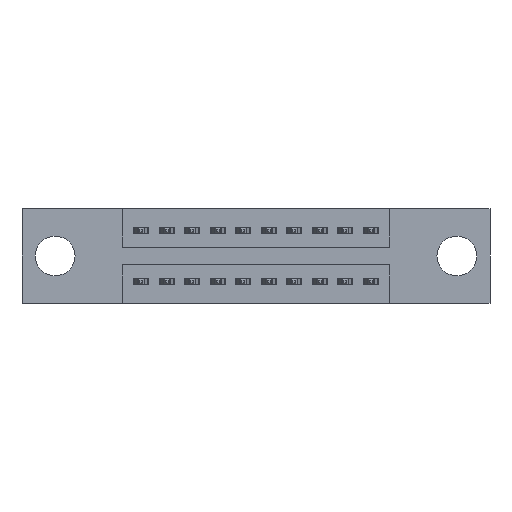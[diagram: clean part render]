
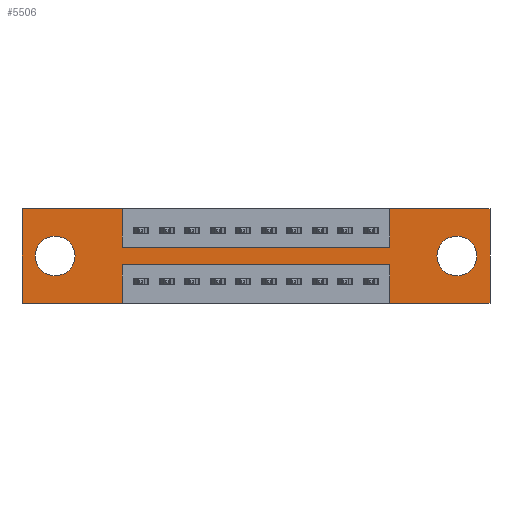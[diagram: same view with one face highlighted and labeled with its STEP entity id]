
A CAD part, front view. The second image highlights one B-rep face of the part: STEP entity #5506.
In plain terms, the highlighted planar face has unit normal (0, -1, 0).
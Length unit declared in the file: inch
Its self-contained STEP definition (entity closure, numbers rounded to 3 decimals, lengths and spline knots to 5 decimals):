
#204 = VERTEX_POINT ( 'NONE', #6562 ) ;
#367 = EDGE_LOOP ( 'NONE', ( #8075, #10543, #10820, #991, #1277, #11371, #1578, #11629, #4822, #7326, #10103, #7926 ) ) ;
#392 = VERTEX_POINT ( 'NONE', #11433 ) ;
#445 = EDGE_CURVE ( 'NONE', #9873, #9577, #7534, .T. ) ;
#560 = VERTEX_POINT ( 'NONE', #6616 ) ;
#700 = EDGE_CURVE ( 'NONE', #11317, #5010, #3963, .T. ) ;
#730 = VECTOR ( 'NONE', #9499, 39.37008 ) ;
#809 = DIRECTION ( 'NONE',  ( 1., 0., 0. ) ) ;
#852 = LINE ( 'NONE', #5624, #5449 ) ;
#991 = ORIENTED_EDGE ( 'NONE', *, *, #1927, .F. ) ;
#1004 = CIRCLE ( 'NONE', #9841, 0.078 ) ;
#1061 = VERTEX_POINT ( 'NONE', #1727 ) ;
#1115 = FACE_OUTER_BOUND ( 'NONE', #367, .T. ) ;
#1277 = ORIENTED_EDGE ( 'NONE', *, *, #700, .F. ) ;
#1292 = CARTESIAN_POINT ( 'NONE',  ( 1.705, 0., -0.185 ) ) ;
#1464 = VECTOR ( 'NONE', #4705, 39.37008 ) ;
#1578 = ORIENTED_EDGE ( 'NONE', *, *, #9920, .F. ) ;
#1727 = CARTESIAN_POINT ( 'NONE',  ( 1.4425, 0., -0.22 ) ) ;
#1927 = EDGE_CURVE ( 'NONE', #5010, #10494, #2683, .T. ) ;
#2093 = DIRECTION ( 'NONE',  ( -1., 0., 0. ) ) ;
#2102 = LINE ( 'NONE', #11151, #9720 ) ;
#2285 = DIRECTION ( 'NONE',  ( 0., 0., -1. ) ) ;
#2384 = CARTESIAN_POINT ( 'NONE',  ( 1.705, 0., -0.185 ) ) ;
#2396 = EDGE_CURVE ( 'NONE', #2643, #392, #3286, .T. ) ;
#2584 = AXIS2_PLACEMENT_3D ( 'NONE', #8527, #2786, #9447 ) ;
#2643 = VERTEX_POINT ( 'NONE', #4557 ) ;
#2674 = CARTESIAN_POINT ( 'NONE',  ( 1.705, 0., -0.263 ) ) ;
#2683 = LINE ( 'NONE', #3256, #9992 ) ;
#2703 = EDGE_CURVE ( 'NONE', #204, #11317, #852, .T. ) ;
#2755 = CARTESIAN_POINT ( 'NONE',  ( 1.4425, 0., 0. ) ) ;
#2786 = DIRECTION ( 'NONE',  ( 0., 1., 0. ) ) ;
#2929 = EDGE_LOOP ( 'NONE', ( #11505, #4972 ) ) ;
#3009 = EDGE_CURVE ( 'NONE', #3177, #2643, #7175, .T. ) ;
#3096 = CARTESIAN_POINT ( 'NONE',  ( 0.3925, 0., 0. ) ) ;
#3177 = VERTEX_POINT ( 'NONE', #7759 ) ;
#3256 = CARTESIAN_POINT ( 'NONE',  ( 0., 0., -0.37 ) ) ;
#3286 = LINE ( 'NONE', #3421, #8969 ) ;
#3310 = LINE ( 'NONE', #3833, #730 ) ;
#3341 = LINE ( 'NONE', #4821, #8158 ) ;
#3421 = CARTESIAN_POINT ( 'NONE',  ( 0.3925, 0., -0.15 ) ) ;
#3685 = EDGE_LOOP ( 'NONE', ( #10675, #8504 ) ) ;
#3833 = CARTESIAN_POINT ( 'NONE',  ( 0.3925, 0., -0.22 ) ) ;
#3906 = CARTESIAN_POINT ( 'NONE',  ( 0., 0., 0. ) ) ;
#3956 = DIRECTION ( 'NONE',  ( 0., 0., -1. ) ) ;
#3959 = CARTESIAN_POINT ( 'NONE',  ( 1.4425, 0., -0.37 ) ) ;
#3963 = LINE ( 'NONE', #12125, #8704 ) ;
#4406 = AXIS2_PLACEMENT_3D ( 'NONE', #11076, #5517, #11918 ) ;
#4557 = CARTESIAN_POINT ( 'NONE',  ( 0.3925, 0., -0.15 ) ) ;
#4592 = VERTEX_POINT ( 'NONE', #5928 ) ;
#4624 = DIRECTION ( 'NONE',  ( 0., 0., -1. ) ) ;
#4677 = VECTOR ( 'NONE', #7447, 39.37008 ) ;
#4703 = CARTESIAN_POINT ( 'NONE',  ( 0.13, 0., -0.107 ) ) ;
#4704 = VECTOR ( 'NONE', #6437, 39.37008 ) ;
#4705 = DIRECTION ( 'NONE',  ( 0., 0., 1. ) ) ;
#4821 = CARTESIAN_POINT ( 'NONE',  ( 0., 0., 0. ) ) ;
#4822 = ORIENTED_EDGE ( 'NONE', *, *, #3009, .F. ) ;
#4892 = DIRECTION ( 'NONE',  ( 1., 0., 0. ) ) ;
#4972 = ORIENTED_EDGE ( 'NONE', *, *, #11687, .T. ) ;
#5010 = VERTEX_POINT ( 'NONE', #9702 ) ;
#5084 = CARTESIAN_POINT ( 'NONE',  ( 0., 0., -0.37 ) ) ;
#5131 = AXIS2_PLACEMENT_3D ( 'NONE', #2384, #7314, #8332 ) ;
#5449 = VECTOR ( 'NONE', #8580, 39.37008 ) ;
#5506 = ADVANCED_FACE ( 'NONE', ( #6011, #6299, #1115 ), #6563, .T. ) ;
#5517 = DIRECTION ( 'NONE',  ( 0., 1., 0. ) ) ;
#5624 = CARTESIAN_POINT ( 'NONE',  ( 0., 0., 0. ) ) ;
#5670 = DIRECTION ( 'NONE',  ( 0., 0., -1. ) ) ;
#5835 = DIRECTION ( 'NONE',  ( 0., 0., 1. ) ) ;
#5928 = CARTESIAN_POINT ( 'NONE',  ( 0.3925, 0., -0.37 ) ) ;
#5969 = AXIS2_PLACEMENT_3D ( 'NONE', #9381, #11222, #5670 ) ;
#6006 = EDGE_CURVE ( 'NONE', #10494, #1061, #6700, .T. ) ;
#6011 = FACE_BOUND ( 'NONE', #3685, .T. ) ;
#6077 = LINE ( 'NONE', #2755, #1464 ) ;
#6299 = FACE_BOUND ( 'NONE', #2929, .T. ) ;
#6437 = DIRECTION ( 'NONE',  ( -1., 0., 0. ) ) ;
#6458 = CIRCLE ( 'NONE', #2584, 0.078 ) ;
#6562 = CARTESIAN_POINT ( 'NONE',  ( 1.4425, 0., 0. ) ) ;
#6563 = PLANE ( 'NONE',  #5969 ) ;
#6616 = CARTESIAN_POINT ( 'NONE',  ( 0.3925, 0., -0.22 ) ) ;
#6700 = LINE ( 'NONE', #3959, #11595 ) ;
#7100 = EDGE_CURVE ( 'NONE', #10215, #11099, #3341, .T. ) ;
#7175 = LINE ( 'NONE', #3096, #4677 ) ;
#7209 = CARTESIAN_POINT ( 'NONE',  ( 1.4425, 0., -0.37 ) ) ;
#7314 = DIRECTION ( 'NONE',  ( 0., 1., 0. ) ) ;
#7326 = ORIENTED_EDGE ( 'NONE', *, *, #7672, .F. ) ;
#7447 = DIRECTION ( 'NONE',  ( 0., 0., -1. ) ) ;
#7534 = CIRCLE ( 'NONE', #5131, 0.078 ) ;
#7672 = EDGE_CURVE ( 'NONE', #11099, #3177, #11562, .T. ) ;
#7759 = CARTESIAN_POINT ( 'NONE',  ( 0.3925, 0., 0. ) ) ;
#7926 = ORIENTED_EDGE ( 'NONE', *, *, #8879, .F. ) ;
#8047 = DIRECTION ( 'NONE',  ( 0., 1., 0. ) ) ;
#8075 = ORIENTED_EDGE ( 'NONE', *, *, #9830, .F. ) ;
#8158 = VECTOR ( 'NONE', #5835, 39.37008 ) ;
#8248 = VERTEX_POINT ( 'NONE', #4703 ) ;
#8293 = EDGE_CURVE ( 'NONE', #1061, #560, #3310, .T. ) ;
#8332 = DIRECTION ( 'NONE',  ( 0., 0., -1. ) ) ;
#8504 = ORIENTED_EDGE ( 'NONE', *, *, #445, .T. ) ;
#8527 = CARTESIAN_POINT ( 'NONE',  ( 0.13, 0., -0.185 ) ) ;
#8580 = DIRECTION ( 'NONE',  ( 1., 0., 0. ) ) ;
#8704 = VECTOR ( 'NONE', #3956, 39.37008 ) ;
#8776 = CARTESIAN_POINT ( 'NONE',  ( 0., 0., 0. ) ) ;
#8879 = EDGE_CURVE ( 'NONE', #4592, #10215, #9996, .T. ) ;
#8969 = VECTOR ( 'NONE', #809, 39.37008 ) ;
#9162 = VECTOR ( 'NONE', #4892, 39.37008 ) ;
#9381 = CARTESIAN_POINT ( 'NONE',  ( 0., 0., -0.37 ) ) ;
#9447 = DIRECTION ( 'NONE',  ( 0., 0., 1. ) ) ;
#9499 = DIRECTION ( 'NONE',  ( -1., 0., 0. ) ) ;
#9577 = VERTEX_POINT ( 'NONE', #10646 ) ;
#9607 = DIRECTION ( 'NONE',  ( 0., 0., 1. ) ) ;
#9702 = CARTESIAN_POINT ( 'NONE',  ( 1.835, 0., -0.37 ) ) ;
#9720 = VECTOR ( 'NONE', #4624, 39.37008 ) ;
#9757 = EDGE_CURVE ( 'NONE', #8248, #10001, #10010, .T. ) ;
#9830 = EDGE_CURVE ( 'NONE', #560, #4592, #2102, .T. ) ;
#9841 = AXIS2_PLACEMENT_3D ( 'NONE', #1292, #8047, #2285 ) ;
#9873 = VERTEX_POINT ( 'NONE', #2674 ) ;
#9920 = EDGE_CURVE ( 'NONE', #392, #204, #6077, .T. ) ;
#9992 = VECTOR ( 'NONE', #2093, 39.37008 ) ;
#9996 = LINE ( 'NONE', #11056, #4704 ) ;
#10001 = VERTEX_POINT ( 'NONE', #10442 ) ;
#10010 = CIRCLE ( 'NONE', #4406, 0.078 ) ;
#10103 = ORIENTED_EDGE ( 'NONE', *, *, #7100, .F. ) ;
#10215 = VERTEX_POINT ( 'NONE', #5084 ) ;
#10442 = CARTESIAN_POINT ( 'NONE',  ( 0.13, 0., -0.263 ) ) ;
#10494 = VERTEX_POINT ( 'NONE', #7209 ) ;
#10543 = ORIENTED_EDGE ( 'NONE', *, *, #8293, .F. ) ;
#10646 = CARTESIAN_POINT ( 'NONE',  ( 1.705, 0., -0.107 ) ) ;
#10675 = ORIENTED_EDGE ( 'NONE', *, *, #11264, .T. ) ;
#10820 = ORIENTED_EDGE ( 'NONE', *, *, #6006, .F. ) ;
#10835 = CARTESIAN_POINT ( 'NONE',  ( 1.835, 0., 0. ) ) ;
#11056 = CARTESIAN_POINT ( 'NONE',  ( 0., 0., -0.37 ) ) ;
#11076 = CARTESIAN_POINT ( 'NONE',  ( 0.13, 0., -0.185 ) ) ;
#11099 = VERTEX_POINT ( 'NONE', #8776 ) ;
#11151 = CARTESIAN_POINT ( 'NONE',  ( 0.3925, 0., -0.37 ) ) ;
#11222 = DIRECTION ( 'NONE',  ( 0., -1., 0. ) ) ;
#11264 = EDGE_CURVE ( 'NONE', #9577, #9873, #1004, .T. ) ;
#11317 = VERTEX_POINT ( 'NONE', #10835 ) ;
#11371 = ORIENTED_EDGE ( 'NONE', *, *, #2703, .F. ) ;
#11433 = CARTESIAN_POINT ( 'NONE',  ( 1.4425, 0., -0.15 ) ) ;
#11505 = ORIENTED_EDGE ( 'NONE', *, *, #9757, .T. ) ;
#11562 = LINE ( 'NONE', #3906, #9162 ) ;
#11595 = VECTOR ( 'NONE', #9607, 39.37008 ) ;
#11629 = ORIENTED_EDGE ( 'NONE', *, *, #2396, .F. ) ;
#11687 = EDGE_CURVE ( 'NONE', #10001, #8248, #6458, .T. ) ;
#11918 = DIRECTION ( 'NONE',  ( 0., 0., 1. ) ) ;
#12125 = CARTESIAN_POINT ( 'NONE',  ( 1.835, 0., 0. ) ) ;
